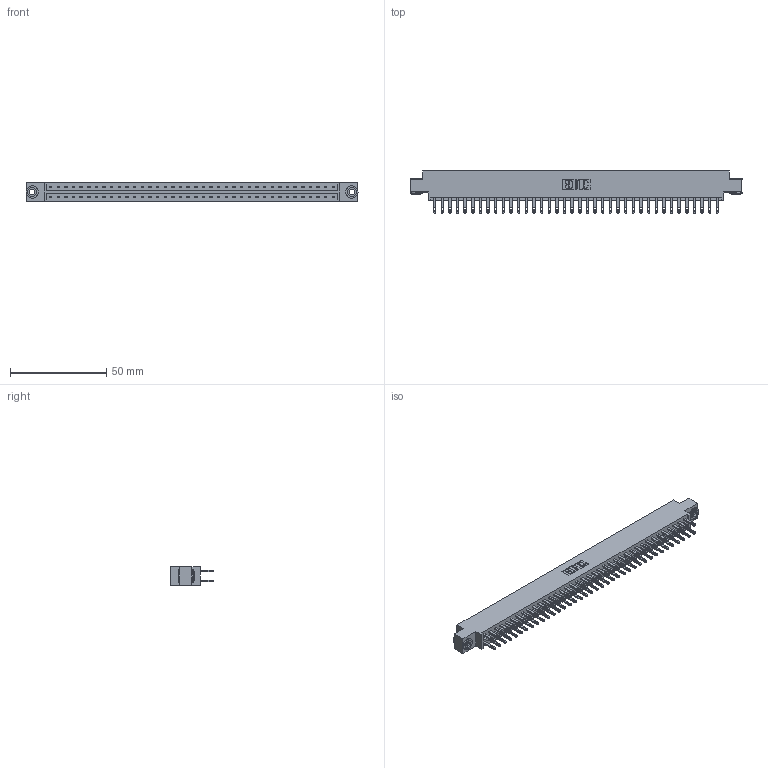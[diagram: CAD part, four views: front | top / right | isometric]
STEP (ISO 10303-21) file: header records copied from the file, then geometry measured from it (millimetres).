
FILE_DESCRIPTION (( 'STEP AP203' ), '1' );
FILE_NAME ('333-076-500-803.STEP', '2018-08-04T22:35:37', ( '' ), ( '' ), 'SwSTEP 2.0', 'SolidWorks 2016', '' );
FILE_SCHEMA (( 'CONFIG_CONTROL_DESIGN' ));
Length unit declared in the file: inch
Products named in the file (4): 333 Part_Offset - .156 Dia - TH; 345-292-001_345-293-100; 345-250-002_345-250-002-102; 333-076-500-803
Assembly tree (79 placements, depth 2):
  333-076-500-803
    333 Part_Offset - .156 Dia - TH
    345-292-001_345-293-100  x76
    345-250-002_345-250-002-102  x2
Bounding box: 172.11 x 21.85 x 9.4 mm (x, y, z)
Volume: 17557.9 mm3; surface area: 21992.9 mm2
Topology: 79 solids, 79 shells, 3804 faces, 11571 edges, 7710 vertices
Faces by surface type: plane 2364, cylinder 1432, cone 8
Entity records: 25676 total; most frequent: CARTESIAN_POINT 4237, ORIENTED_EDGE 4166, DIRECTION 3661, EDGE_CURVE 2083, VECTOR 1927, LINE 1927, VERTEX_POINT 1386, AXIS2_PLACEMENT_3D 867
